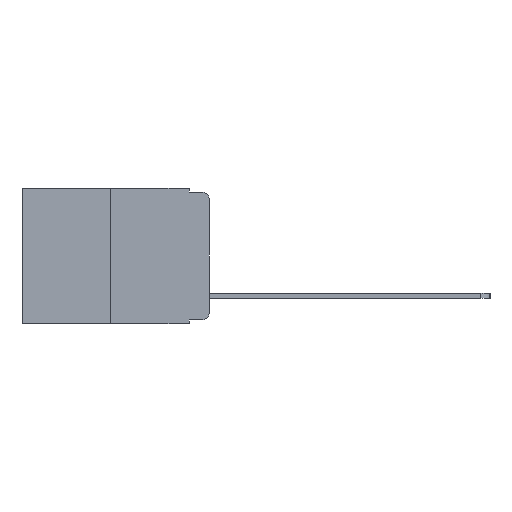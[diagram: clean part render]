
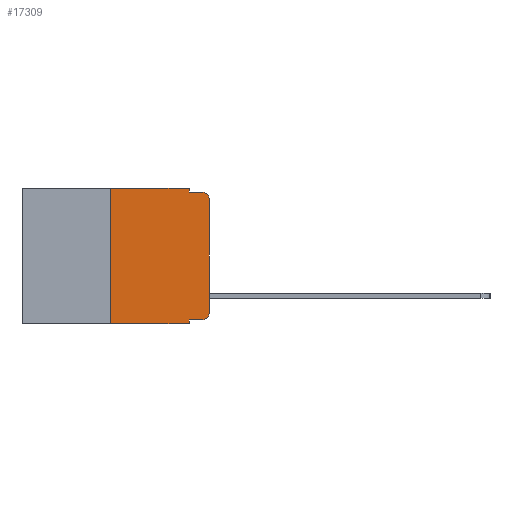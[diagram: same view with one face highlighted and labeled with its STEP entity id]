
A CAD part, left-side view. The second image highlights one B-rep face of the part: STEP entity #17309.
In plain terms, the highlighted planar face has unit normal (-1, 0, 0).
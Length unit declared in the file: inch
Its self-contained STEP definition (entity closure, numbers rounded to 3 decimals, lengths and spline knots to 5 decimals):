
#317 = VECTOR ( 'NONE', #5459, 39.37008 ) ;
#930 = ORIENTED_EDGE ( 'NONE', *, *, #11480, .T. ) ;
#1286 = CARTESIAN_POINT ( 'NONE',  ( 0., 0.25, 0. ) ) ;
#1342 = DIRECTION ( 'NONE',  ( 0., 0., -1. ) ) ;
#1368 = DIRECTION ( 'NONE',  ( -1., 0., 0. ) ) ;
#1384 = CARTESIAN_POINT ( 'NONE',  ( 0., 0.02, -0.313 ) ) ;
#1464 = CARTESIAN_POINT ( 'NONE',  ( 0., 0.02, -0.333 ) ) ;
#1790 = EDGE_LOOP ( 'NONE', ( #16905, #930, #6375, #3957, #10519, #13934, #15768, #10736, #17685, #13718 ) ) ;
#1938 = EDGE_CURVE ( 'NONE', #4113, #8837, #2281, .T. ) ;
#2281 = LINE ( 'NONE', #14985, #17235 ) ;
#2303 = DIRECTION ( 'NONE',  ( 0., 0., 1. ) ) ;
#2767 = CARTESIAN_POINT ( 'NONE',  ( 0., 0.051, -0.01 ) ) ;
#2987 = EDGE_CURVE ( 'NONE', #10123, #15995, #7877, .T. ) ;
#3932 = LINE ( 'NONE', #12931, #14740 ) ;
#3957 = ORIENTED_EDGE ( 'NONE', *, *, #11758, .F. ) ;
#4031 = FACE_OUTER_BOUND ( 'NONE', #1790, .T. ) ;
#4066 = CARTESIAN_POINT ( 'NONE',  ( 0., 0.473, 0. ) ) ;
#4113 = VERTEX_POINT ( 'NONE', #8255 ) ;
#4994 = CARTESIAN_POINT ( 'NONE',  ( 0., 0.25, -0.343 ) ) ;
#5083 = VERTEX_POINT ( 'NONE', #18767 ) ;
#5111 = VERTEX_POINT ( 'NONE', #13101 ) ;
#5459 = DIRECTION ( 'NONE',  ( 0., 0., -1. ) ) ;
#5482 = DIRECTION ( 'NONE',  ( 0., -1., 0. ) ) ;
#5563 = DIRECTION ( 'NONE',  ( 0., 0., -1. ) ) ;
#5808 = CARTESIAN_POINT ( 'NONE',  ( 0., 0., -0.313 ) ) ;
#6206 = CIRCLE ( 'NONE', #15499, 0.02 ) ;
#6239 = DIRECTION ( 'NONE',  ( 0., -1., 0. ) ) ;
#6295 = AXIS2_PLACEMENT_3D ( 'NONE', #1384, #1368, #1342 ) ;
#6336 = DIRECTION ( 'NONE',  ( -1., 0., 0. ) ) ;
#6375 = ORIENTED_EDGE ( 'NONE', *, *, #17937, .F. ) ;
#6474 = VECTOR ( 'NONE', #17792, 39.37008 ) ;
#6646 = CARTESIAN_POINT ( 'NONE',  ( 0., 0., -0.03 ) ) ;
#6944 = LINE ( 'NONE', #16413, #6474 ) ;
#7140 = CARTESIAN_POINT ( 'NONE',  ( 0., 0.051, -0.343 ) ) ;
#7424 = VECTOR ( 'NONE', #8885, 39.37008 ) ;
#7639 = LINE ( 'NONE', #1286, #7424 ) ;
#7759 = CARTESIAN_POINT ( 'NONE',  ( 0., 0.051, -0.333 ) ) ;
#7877 = CIRCLE ( 'NONE', #6295, 0.02 ) ;
#8255 = CARTESIAN_POINT ( 'NONE',  ( 0., 0.051, -0.333 ) ) ;
#8659 = VECTOR ( 'NONE', #2303, 39.37008 ) ;
#8837 = VERTEX_POINT ( 'NONE', #7140 ) ;
#8885 = DIRECTION ( 'NONE',  ( 0., 0., 1. ) ) ;
#8890 = VERTEX_POINT ( 'NONE', #2767 ) ;
#9130 = LINE ( 'NONE', #11336, #8659 ) ;
#9227 = VECTOR ( 'NONE', #11547, 39.37008 ) ;
#10123 = VERTEX_POINT ( 'NONE', #1464 ) ;
#10493 = EDGE_CURVE ( 'NONE', #15995, #12308, #9130, .T. ) ;
#10519 = ORIENTED_EDGE ( 'NONE', *, *, #14116, .F. ) ;
#10736 = ORIENTED_EDGE ( 'NONE', *, *, #1938, .F. ) ;
#11336 = CARTESIAN_POINT ( 'NONE',  ( 0., 0., 0. ) ) ;
#11480 = EDGE_CURVE ( 'NONE', #12308, #5111, #6206, .T. ) ;
#11547 = DIRECTION ( 'NONE',  ( 0., -1., 0. ) ) ;
#11758 = EDGE_CURVE ( 'NONE', #17637, #8890, #16002, .T. ) ;
#11772 = DIRECTION ( 'NONE',  ( 0., 0., -1. ) ) ;
#12041 = LINE ( 'NONE', #7759, #14837 ) ;
#12229 = VERTEX_POINT ( 'NONE', #4994 ) ;
#12308 = VERTEX_POINT ( 'NONE', #6646 ) ;
#12931 = CARTESIAN_POINT ( 'NONE',  ( 0., 0.473, -0.343 ) ) ;
#13101 = CARTESIAN_POINT ( 'NONE',  ( 0., 0.02, -0.01 ) ) ;
#13110 = LINE ( 'NONE', #15653, #9227 ) ;
#13196 = EDGE_CURVE ( 'NONE', #12229, #8837, #3932, .T. ) ;
#13718 = ORIENTED_EDGE ( 'NONE', *, *, #2987, .T. ) ;
#13825 = CARTESIAN_POINT ( 'NONE',  ( 0., 0.051, 0. ) ) ;
#13934 = ORIENTED_EDGE ( 'NONE', *, *, #18856, .F. ) ;
#14116 = EDGE_CURVE ( 'NONE', #5083, #17637, #6944, .T. ) ;
#14203 = AXIS2_PLACEMENT_3D ( 'NONE', #4066, #14378, #5563 ) ;
#14234 = CARTESIAN_POINT ( 'NONE',  ( 0., 0.051, 0. ) ) ;
#14378 = DIRECTION ( 'NONE',  ( 1., 0., 0. ) ) ;
#14740 = VECTOR ( 'NONE', #5482, 39.37008 ) ;
#14837 = VECTOR ( 'NONE', #6239, 39.37008 ) ;
#14985 = CARTESIAN_POINT ( 'NONE',  ( 0., 0.051, 0. ) ) ;
#15048 = CARTESIAN_POINT ( 'NONE',  ( 0., 0.02, -0.03 ) ) ;
#15499 = AXIS2_PLACEMENT_3D ( 'NONE', #15048, #6336, #16368 ) ;
#15653 = CARTESIAN_POINT ( 'NONE',  ( 0., 0.051, -0.01 ) ) ;
#15768 = ORIENTED_EDGE ( 'NONE', *, *, #13196, .T. ) ;
#15995 = VERTEX_POINT ( 'NONE', #5808 ) ;
#16002 = LINE ( 'NONE', #14234, #317 ) ;
#16368 = DIRECTION ( 'NONE',  ( 0., 0., -1. ) ) ;
#16413 = CARTESIAN_POINT ( 'NONE',  ( 0., 0.473, 0. ) ) ;
#16902 = EDGE_CURVE ( 'NONE', #4113, #10123, #12041, .T. ) ;
#16905 = ORIENTED_EDGE ( 'NONE', *, *, #10493, .T. ) ;
#17235 = VECTOR ( 'NONE', #11772, 39.37008 ) ;
#17309 = ADVANCED_FACE ( 'NONE', ( #4031 ), #18382, .F. ) ;
#17637 = VERTEX_POINT ( 'NONE', #13825 ) ;
#17685 = ORIENTED_EDGE ( 'NONE', *, *, #16902, .T. ) ;
#17792 = DIRECTION ( 'NONE',  ( 0., -1., 0. ) ) ;
#17937 = EDGE_CURVE ( 'NONE', #8890, #5111, #13110, .T. ) ;
#18382 = PLANE ( 'NONE',  #14203 ) ;
#18767 = CARTESIAN_POINT ( 'NONE',  ( 0., 0.25, 0. ) ) ;
#18856 = EDGE_CURVE ( 'NONE', #12229, #5083, #7639, .T. ) ;
